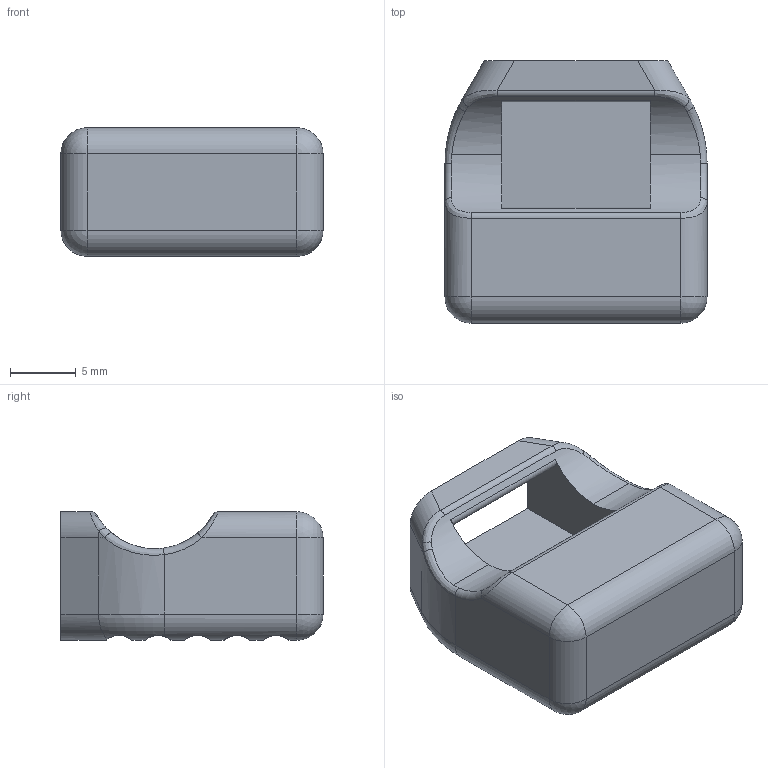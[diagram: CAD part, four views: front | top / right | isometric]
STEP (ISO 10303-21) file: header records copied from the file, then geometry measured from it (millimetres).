
FILE_DESCRIPTION (( 'STEP AP214' ), '1' );
FILE_NAME ('Mag_Release_Button_V1.STEP', '2025-07-07T03:52:44', ( '' ), ( '' ), 'SwSTEP 2.0', 'SolidWorks 2020', '' );
FILE_SCHEMA (( 'AUTOMOTIVE_DESIGN' ));
Length unit declared in the file: millimetre
Products named in the file (1): Mag_Release_Button_V1
Bounding box: 20 x 20 x 9.8 mm (x, y, z)
Volume: 2595.9 mm3; surface area: 1600.1 mm2
Topology: 1 solids, 1 shells, 63 faces, 160 edges, 94 vertices
Faces by surface type: cylinder 25, plane 20, bspline 8, torus 6, sphere 4
Entity records: 2352 total; most frequent: CARTESIAN_POINT 898, ORIENTED_EDGE 312, DIRECTION 280, EDGE_CURVE 156, AXIS2_PLACEMENT_3D 104, VERTEX_POINT 94, VECTOR 72, LINE 72
